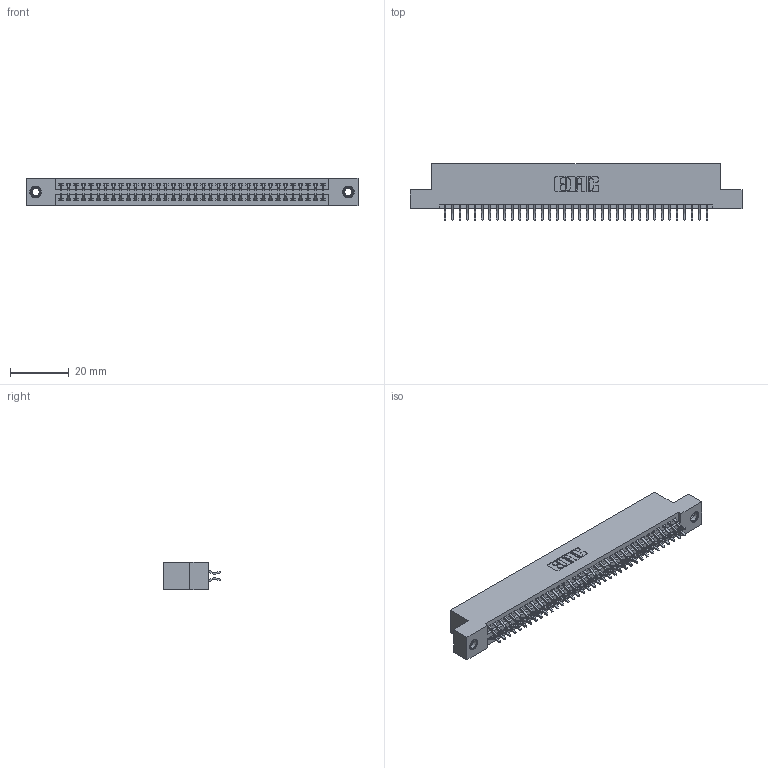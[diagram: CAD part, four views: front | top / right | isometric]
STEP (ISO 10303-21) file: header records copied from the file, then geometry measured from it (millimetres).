
FILE_DESCRIPTION (( 'STEP AP203' ), '1' );
FILE_NAME ('345-072-556-207.STEP', '2018-10-02T08:46:55', ( '' ), ( '' ), 'SwSTEP 2.0', 'SolidWorks 2016', '' );
FILE_SCHEMA (( 'CONFIG_CONTROL_DESIGN' ));
Length unit declared in the file: inch
Products named in the file (4): 345-250-001_345-250-005-103; 345-292-001_556 Tail; 345 Part_Flush Mounting Lugs - 0.156 Dia-TI; 345-072-556-207
Assembly tree (75 placements, depth 2):
  345-072-556-207
    345 Part_Flush Mounting Lugs - 0.156 Dia-TI
    345-292-001_556 Tail  x72
    345-250-001_345-250-005-103  x2
Bounding box: 112.65 x 19.24 x 9.4 mm (x, y, z)
Volume: 10870.8 mm3; surface area: 15917.5 mm2
Topology: 75 solids, 75 shells, 4218 faces, 12501 edges, 8230 vertices
Faces by surface type: plane 2776, cylinder 1426, cone 12, torus 4
Entity records: 30460 total; most frequent: CARTESIAN_POINT 5107, ORIENTED_EDGE 5022, DIRECTION 4525, EDGE_CURVE 2511, LINE 2207, VECTOR 2207, VERTEX_POINT 1668, AXIS2_PLACEMENT_3D 1159
